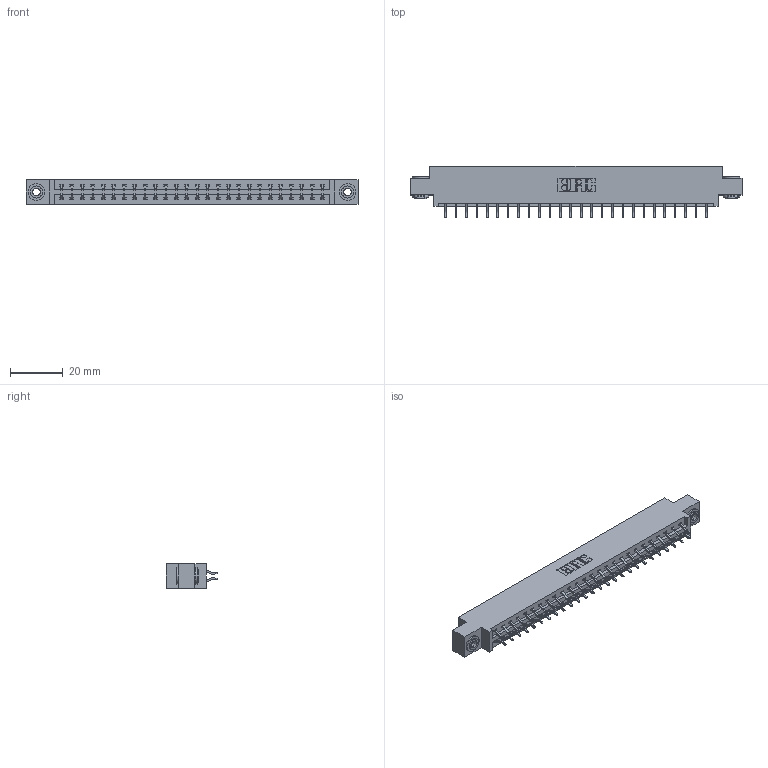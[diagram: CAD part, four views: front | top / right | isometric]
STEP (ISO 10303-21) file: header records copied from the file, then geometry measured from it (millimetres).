
FILE_DESCRIPTION (( 'STEP AP203' ), '1' );
FILE_NAME ('337-052-556-803.STEP', '2018-08-09T23:26:43', ( '' ), ( '' ), 'SwSTEP 2.0', 'SolidWorks 2016', '' );
FILE_SCHEMA (( 'CONFIG_CONTROL_DESIGN' ));
Length unit declared in the file: inch
Products named in the file (4): 337-052-556-803; 337 Part_0.170 Offset - 0.156 Dia-TH; 345-292-001_556 Tail; 345-250-002_345-250-002-102
Assembly tree (55 placements, depth 2):
  337-052-556-803
    337 Part_0.170 Offset - 0.156 Dia-TH
    345-292-001_556 Tail  x52
    345-250-002_345-250-002-102  x2
Bounding box: 126.03 x 19.57 x 9.4 mm (x, y, z)
Volume: 12969.4 mm3; surface area: 14783.9 mm2
Topology: 55 solids, 55 shells, 3276 faces, 9707 edges, 6398 vertices
Faces by surface type: plane 2268, cylinder 1000, cone 8
Entity records: 23230 total; most frequent: CARTESIAN_POINT 3917, ORIENTED_EDGE 3834, DIRECTION 3383, EDGE_CURVE 1917, LINE 1757, VECTOR 1757, VERTEX_POINT 1274, AXIS2_PLACEMENT_3D 813
